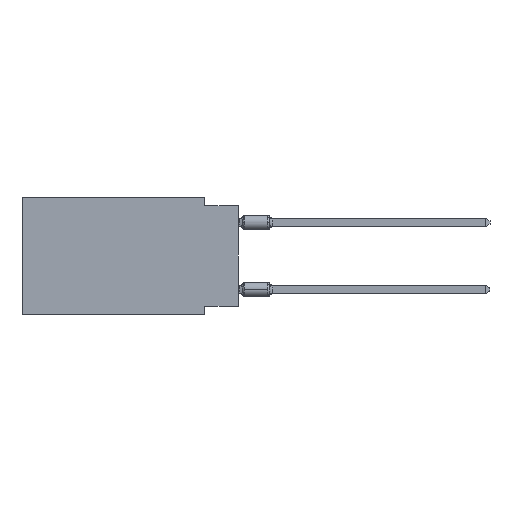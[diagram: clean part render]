
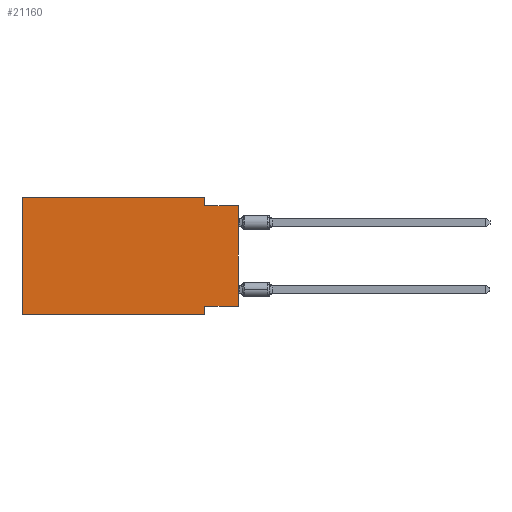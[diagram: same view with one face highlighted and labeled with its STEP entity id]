
A CAD part, left-side view. The second image highlights one B-rep face of the part: STEP entity #21160.
In plain terms, the highlighted planar face has unit normal (-1, 0, 0).
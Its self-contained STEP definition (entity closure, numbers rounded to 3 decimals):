
#51 = FACE_OUTER_BOUND ( 'NONE', #5836, .T. ) ;
#508 = DIRECTION ( 'NONE',  ( 0., -1., 0. ) ) ;
#688 = VECTOR ( 'NONE', #3330, 1000. ) ;
#752 = LINE ( 'NONE', #16957, #13126 ) ;
#1586 = EDGE_CURVE ( 'NONE', #28021, #2373, #13435, .T. ) ;
#1747 = ORIENTED_EDGE ( 'NONE', *, *, #7003, .F. ) ;
#2280 = VERTEX_POINT ( 'NONE', #25737 ) ;
#2373 = VERTEX_POINT ( 'NONE', #20194 ) ;
#3205 = ORIENTED_EDGE ( 'NONE', *, *, #6426, .F. ) ;
#3237 = CARTESIAN_POINT ( 'NONE',  ( 0., 2.54, -8.255 ) ) ;
#3330 = DIRECTION ( 'NONE',  ( 0., 0., 1. ) ) ;
#3798 = CARTESIAN_POINT ( 'NONE',  ( 0., 16.383, -8.89 ) ) ;
#3914 = ORIENTED_EDGE ( 'NONE', *, *, #21184, .F. ) ;
#3923 = VECTOR ( 'NONE', #22743, 1000. ) ;
#4795 = CARTESIAN_POINT ( 'NONE',  ( 0., 16.383, 0. ) ) ;
#5244 = CARTESIAN_POINT ( 'NONE',  ( 0., 16.383, 0. ) ) ;
#5836 = EDGE_LOOP ( 'NONE', ( #12114, #20748, #3914, #1747, #3205, #14135, #14414, #27822 ) ) ;
#6348 = LINE ( 'NONE', #24509, #20626 ) ;
#6426 = EDGE_CURVE ( 'NONE', #28021, #2280, #6348, .T. ) ;
#6458 = LINE ( 'NONE', #29231, #12280 ) ;
#6603 = PLANE ( 'NONE',  #8498 ) ;
#6655 = VERTEX_POINT ( 'NONE', #19565 ) ;
#6786 = DIRECTION ( 'NONE',  ( 0., 0., 1. ) ) ;
#7003 = EDGE_CURVE ( 'NONE', #2280, #22081, #16255, .T. ) ;
#8253 = DIRECTION ( 'NONE',  ( 0., -1., 0. ) ) ;
#8498 = AXIS2_PLACEMENT_3D ( 'NONE', #4795, #15971, #22960 ) ;
#8774 = CARTESIAN_POINT ( 'NONE',  ( 0., 16.383, -8.89 ) ) ;
#11859 = EDGE_CURVE ( 'NONE', #19405, #23292, #25791, .T. ) ;
#12114 = ORIENTED_EDGE ( 'NONE', *, *, #11859, .T. ) ;
#12280 = VECTOR ( 'NONE', #25059, 1000. ) ;
#13126 = VECTOR ( 'NONE', #27839, 1000. ) ;
#13435 = LINE ( 'NONE', #3798, #25372 ) ;
#14135 = ORIENTED_EDGE ( 'NONE', *, *, #1586, .T. ) ;
#14414 = ORIENTED_EDGE ( 'NONE', *, *, #28446, .F. ) ;
#15156 = EDGE_CURVE ( 'NONE', #19405, #20564, #752, .T. ) ;
#15432 = CARTESIAN_POINT ( 'NONE',  ( 0., 2.54, -8.89 ) ) ;
#15971 = DIRECTION ( 'NONE',  ( 1., 0., 0. ) ) ;
#16162 = LINE ( 'NONE', #25112, #25269 ) ;
#16255 = LINE ( 'NONE', #5244, #21117 ) ;
#16957 = CARTESIAN_POINT ( 'NONE',  ( 0., 0., -8.255 ) ) ;
#18645 = CARTESIAN_POINT ( 'NONE',  ( 0., 0., 0. ) ) ;
#19405 = VERTEX_POINT ( 'NONE', #27401 ) ;
#19565 = CARTESIAN_POINT ( 'NONE',  ( 0., 2.54, -0.635 ) ) ;
#19917 = LINE ( 'NONE', #15432, #3923 ) ;
#20194 = CARTESIAN_POINT ( 'NONE',  ( 0., 2.54, -8.89 ) ) ;
#20564 = VERTEX_POINT ( 'NONE', #3237 ) ;
#20626 = VECTOR ( 'NONE', #6786, 1000. ) ;
#20645 = DIRECTION ( 'NONE',  ( 0., -1., 0. ) ) ;
#20748 = ORIENTED_EDGE ( 'NONE', *, *, #26954, .F. ) ;
#21117 = VECTOR ( 'NONE', #508, 1000. ) ;
#21160 = ADVANCED_FACE ( 'NONE', ( #51 ), #6603, .F. ) ;
#21184 = EDGE_CURVE ( 'NONE', #22081, #6655, #6458, .T. ) ;
#22081 = VERTEX_POINT ( 'NONE', #23429 ) ;
#22743 = DIRECTION ( 'NONE',  ( 0., 0., -1. ) ) ;
#22960 = DIRECTION ( 'NONE',  ( 0., 0., -1. ) ) ;
#23292 = VERTEX_POINT ( 'NONE', #26283 ) ;
#23429 = CARTESIAN_POINT ( 'NONE',  ( 0., 2.54, 0. ) ) ;
#24509 = CARTESIAN_POINT ( 'NONE',  ( 0., 16.383, 0. ) ) ;
#25059 = DIRECTION ( 'NONE',  ( 0., 0., -1. ) ) ;
#25112 = CARTESIAN_POINT ( 'NONE',  ( 0., 0., -0.635 ) ) ;
#25269 = VECTOR ( 'NONE', #20645, 1000. ) ;
#25372 = VECTOR ( 'NONE', #8253, 1000. ) ;
#25737 = CARTESIAN_POINT ( 'NONE',  ( 0., 16.383, 0. ) ) ;
#25791 = LINE ( 'NONE', #18645, #688 ) ;
#26283 = CARTESIAN_POINT ( 'NONE',  ( 0., 0., -0.635 ) ) ;
#26954 = EDGE_CURVE ( 'NONE', #6655, #23292, #16162, .T. ) ;
#27401 = CARTESIAN_POINT ( 'NONE',  ( 0., 0., -8.255 ) ) ;
#27822 = ORIENTED_EDGE ( 'NONE', *, *, #15156, .F. ) ;
#27839 = DIRECTION ( 'NONE',  ( 0., 1., 0. ) ) ;
#28021 = VERTEX_POINT ( 'NONE', #8774 ) ;
#28446 = EDGE_CURVE ( 'NONE', #20564, #2373, #19917, .T. ) ;
#29231 = CARTESIAN_POINT ( 'NONE',  ( 0., 2.54, 0. ) ) ;
